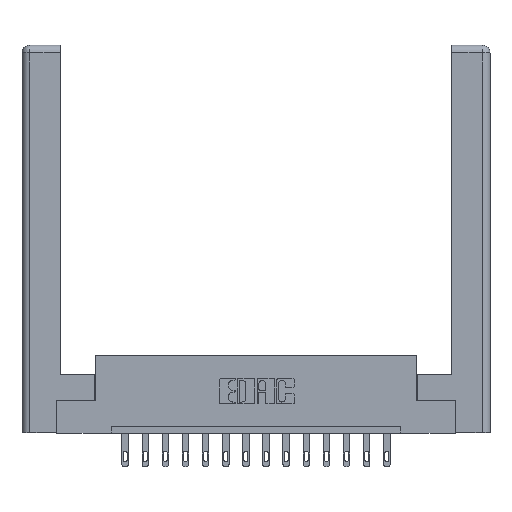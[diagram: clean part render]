
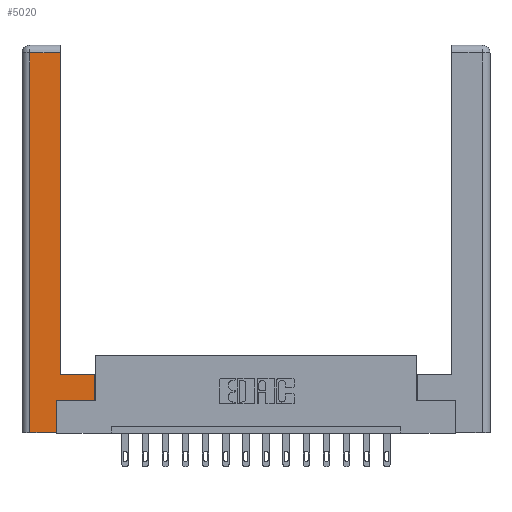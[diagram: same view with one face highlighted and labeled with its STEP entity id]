
A CAD part, top view. The second image highlights one B-rep face of the part: STEP entity #5020.
In plain terms, the highlighted planar face has unit normal (0, 0, 1).
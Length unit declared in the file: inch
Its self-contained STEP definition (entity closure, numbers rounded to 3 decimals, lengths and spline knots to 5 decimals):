
#33 = CARTESIAN_POINT ( 'NONE',  ( 0., 0., 0. ) ) ;
#585 = EDGE_CURVE ( 'NONE', #3327, #4843, #7836, .T. ) ;
#1245 = VECTOR ( 'NONE', #5191, 39.37008 ) ;
#1602 = AXIS2_PLACEMENT_3D ( 'NONE', #33, #14135, #9213 ) ;
#1830 = ORIENTED_EDGE ( 'NONE', *, *, #5757, .T. ) ;
#2024 = EDGE_CURVE ( 'NONE', #11083, #7982, #12834, .T. ) ;
#2492 = ORIENTED_EDGE ( 'NONE', *, *, #11256, .T. ) ;
#2568 = ORIENTED_EDGE ( 'NONE', *, *, #2024, .T. ) ;
#2850 = ORIENTED_EDGE ( 'NONE', *, *, #11631, .T. ) ;
#3172 = VERTEX_POINT ( 'NONE', #6011 ) ;
#3204 = LINE ( 'NONE', #7718, #12590 ) ;
#3327 = VERTEX_POINT ( 'NONE', #5880 ) ;
#3455 = EDGE_CURVE ( 'NONE', #7982, #3172, #12768, .T. ) ;
#3476 = LINE ( 'NONE', #4935, #11065 ) ;
#3940 = DIRECTION ( 'NONE',  ( 0., 1., 0. ) ) ;
#4166 = CARTESIAN_POINT ( 'NONE',  ( 0.0615, 2.94, 0. ) ) ;
#4305 = LINE ( 'NONE', #10348, #4875 ) ;
#4843 = VERTEX_POINT ( 'NONE', #13367 ) ;
#4875 = VECTOR ( 'NONE', #14228, 39.37008 ) ;
#4935 = CARTESIAN_POINT ( 'NONE',  ( 0.295, 0.45, 0. ) ) ;
#5020 = ADVANCED_FACE ( 'NONE', ( #11293 ), #12929, .F. ) ;
#5191 = DIRECTION ( 'NONE',  ( 0., 1., 0. ) ) ;
#5757 = EDGE_CURVE ( 'NONE', #15186, #11083, #3476, .T. ) ;
#5880 = CARTESIAN_POINT ( 'NONE',  ( 0.0615, 0., 0. ) ) ;
#6011 = CARTESIAN_POINT ( 'NONE',  ( 0.0615, 2.94, 0. ) ) ;
#6773 = CARTESIAN_POINT ( 'NONE',  ( 0.265, 0., 0. ) ) ;
#7382 = VECTOR ( 'NONE', #15709, 39.37008 ) ;
#7718 = CARTESIAN_POINT ( 'NONE',  ( 0.265, 0.245, 0. ) ) ;
#7810 = ORIENTED_EDGE ( 'NONE', *, *, #585, .T. ) ;
#7836 = LINE ( 'NONE', #6773, #12007 ) ;
#7842 = VERTEX_POINT ( 'NONE', #14034 ) ;
#7982 = VERTEX_POINT ( 'NONE', #10436 ) ;
#8088 = ORIENTED_EDGE ( 'NONE', *, *, #12660, .T. ) ;
#8627 = CARTESIAN_POINT ( 'NONE',  ( 0.565, 0.245, 0. ) ) ;
#8668 = DIRECTION ( 'NONE',  ( 0., 1., 0. ) ) ;
#8847 = LINE ( 'NONE', #15222, #11606 ) ;
#9008 = EDGE_LOOP ( 'NONE', ( #2568, #12849, #8088, #7810, #2850, #13666, #2492, #1830 ) ) ;
#9043 = CARTESIAN_POINT ( 'NONE',  ( 0.295, 0.45, 0. ) ) ;
#9114 = CARTESIAN_POINT ( 'NONE',  ( 0.295, 3., 0. ) ) ;
#9115 = DIRECTION ( 'NONE',  ( -1., 0., 0. ) ) ;
#9185 = LINE ( 'NONE', #13292, #7382 ) ;
#9213 = DIRECTION ( 'NONE',  ( -1., 0., 0. ) ) ;
#10267 = VERTEX_POINT ( 'NONE', #8627 ) ;
#10348 = CARTESIAN_POINT ( 'NONE',  ( 0.565, 0.245, 0. ) ) ;
#10436 = CARTESIAN_POINT ( 'NONE',  ( 0.295, 2.94, 0. ) ) ;
#11065 = VECTOR ( 'NONE', #12505, 39.37008 ) ;
#11083 = VERTEX_POINT ( 'NONE', #9043 ) ;
#11256 = EDGE_CURVE ( 'NONE', #10267, #15186, #8847, .T. ) ;
#11293 = FACE_OUTER_BOUND ( 'NONE', #9008, .T. ) ;
#11606 = VECTOR ( 'NONE', #8668, 39.37008 ) ;
#11631 = EDGE_CURVE ( 'NONE', #4843, #7842, #3204, .T. ) ;
#12007 = VECTOR ( 'NONE', #15596, 39.37008 ) ;
#12070 = CARTESIAN_POINT ( 'NONE',  ( 0.565, 0.45, 0. ) ) ;
#12505 = DIRECTION ( 'NONE',  ( -1., 0., 0. ) ) ;
#12590 = VECTOR ( 'NONE', #3940, 39.37008 ) ;
#12660 = EDGE_CURVE ( 'NONE', #3172, #3327, #9185, .T. ) ;
#12768 = LINE ( 'NONE', #4166, #13156 ) ;
#12834 = LINE ( 'NONE', #9114, #1245 ) ;
#12849 = ORIENTED_EDGE ( 'NONE', *, *, #3455, .T. ) ;
#12929 = PLANE ( 'NONE',  #1602 ) ;
#13156 = VECTOR ( 'NONE', #9115, 39.37008 ) ;
#13292 = CARTESIAN_POINT ( 'NONE',  ( 0.0615, 0., 0. ) ) ;
#13367 = CARTESIAN_POINT ( 'NONE',  ( 0.265, 0., 0. ) ) ;
#13666 = ORIENTED_EDGE ( 'NONE', *, *, #14361, .T. ) ;
#14034 = CARTESIAN_POINT ( 'NONE',  ( 0.265, 0.245, 0. ) ) ;
#14135 = DIRECTION ( 'NONE',  ( 0., 0., -1. ) ) ;
#14228 = DIRECTION ( 'NONE',  ( 1., 0., 0. ) ) ;
#14361 = EDGE_CURVE ( 'NONE', #7842, #10267, #4305, .T. ) ;
#15186 = VERTEX_POINT ( 'NONE', #12070 ) ;
#15222 = CARTESIAN_POINT ( 'NONE',  ( 0.565, 0.45, 0. ) ) ;
#15596 = DIRECTION ( 'NONE',  ( 1., 0., 0. ) ) ;
#15709 = DIRECTION ( 'NONE',  ( 0., -1., 0. ) ) ;
